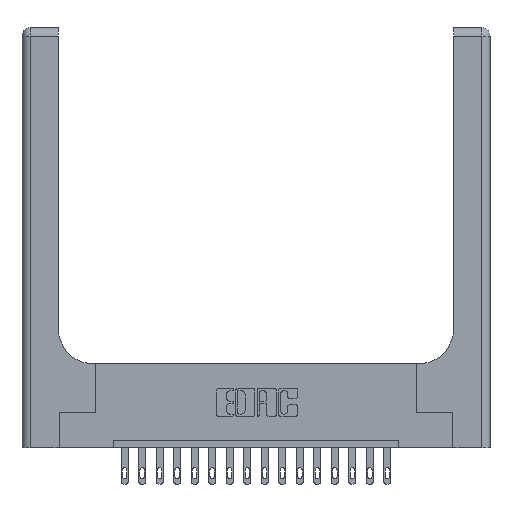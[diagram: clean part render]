
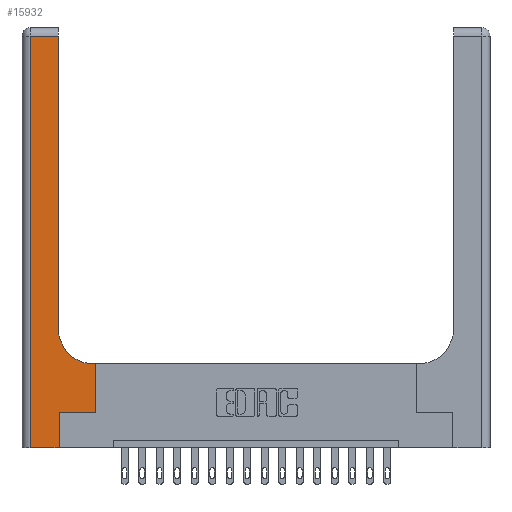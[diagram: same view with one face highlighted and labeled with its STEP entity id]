
A CAD part, top view. The second image highlights one B-rep face of the part: STEP entity #15932.
In plain terms, the highlighted planar face has unit normal (0, 0, 1).
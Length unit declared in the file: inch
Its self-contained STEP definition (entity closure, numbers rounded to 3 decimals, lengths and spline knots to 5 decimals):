
#369 = VERTEX_POINT ( 'NONE', #13812 ) ;
#607 = CARTESIAN_POINT ( 'NONE',  ( 0.265, 0., 0.37 ) ) ;
#915 = VERTEX_POINT ( 'NONE', #9989 ) ;
#1309 = ORIENTED_EDGE ( 'NONE', *, *, #14490, .T. ) ;
#1994 = ORIENTED_EDGE ( 'NONE', *, *, #11978, .T. ) ;
#2414 = CARTESIAN_POINT ( 'NONE',  ( 0., 0., 0.37 ) ) ;
#2613 = VECTOR ( 'NONE', #3500, 39.37008 ) ;
#2908 = CARTESIAN_POINT ( 'NONE',  ( 0.265, 0.25, 0.37 ) ) ;
#2910 = DIRECTION ( 'NONE',  ( -1., 0., 0. ) ) ;
#2995 = VECTOR ( 'NONE', #15745, 39.37008 ) ;
#3332 = VERTEX_POINT ( 'NONE', #2908 ) ;
#3500 = DIRECTION ( 'NONE',  ( 1., 0., 0. ) ) ;
#3819 = LINE ( 'NONE', #12931, #16056 ) ;
#3874 = CARTESIAN_POINT ( 'NONE',  ( 0.26, 3., 0.37 ) ) ;
#4106 = DIRECTION ( 'NONE',  ( 0., -1., 0. ) ) ;
#4144 = CARTESIAN_POINT ( 'NONE',  ( 0.528, 0.6, 0.37 ) ) ;
#4462 = ORIENTED_EDGE ( 'NONE', *, *, #13553, .T. ) ;
#5079 = AXIS2_PLACEMENT_3D ( 'NONE', #10097, #7033, #2910 ) ;
#6234 = CARTESIAN_POINT ( 'NONE',  ( 0., 2.94, 0.37 ) ) ;
#6255 = VERTEX_POINT ( 'NONE', #17951 ) ;
#6872 = VECTOR ( 'NONE', #14143, 39.37008 ) ;
#6894 = LINE ( 'NONE', #12766, #10780 ) ;
#6997 = CARTESIAN_POINT ( 'NONE',  ( 0.06, 2.94, 0.37 ) ) ;
#7033 = DIRECTION ( 'NONE',  ( 0., 0., -1. ) ) ;
#7775 = ORIENTED_EDGE ( 'NONE', *, *, #14515, .T. ) ;
#8270 = CARTESIAN_POINT ( 'NONE',  ( 0.51, 0.85, 0.37 ) ) ;
#8745 = PLANE ( 'NONE',  #5079 ) ;
#8755 = VECTOR ( 'NONE', #15331, 39.37008 ) ;
#8952 = EDGE_CURVE ( 'NONE', #15361, #11487, #13760, .T. ) ;
#9429 = ORIENTED_EDGE ( 'NONE', *, *, #8952, .T. ) ;
#9489 = ORIENTED_EDGE ( 'NONE', *, *, #10337, .T. ) ;
#9832 = CARTESIAN_POINT ( 'NONE',  ( 0.528, 0.25, 0.37 ) ) ;
#9989 = CARTESIAN_POINT ( 'NONE',  ( 0.26, 0.85, 0.37 ) ) ;
#10097 = CARTESIAN_POINT ( 'NONE',  ( 0., 3., 0.37 ) ) ;
#10206 = VECTOR ( 'NONE', #18162, 39.37008 ) ;
#10337 = EDGE_CURVE ( 'NONE', #6255, #14949, #17002, .T. ) ;
#10780 = VECTOR ( 'NONE', #18622, 39.37008 ) ;
#11164 = LINE ( 'NONE', #3874, #6872 ) ;
#11422 = EDGE_CURVE ( 'NONE', #14949, #3332, #18356, .T. ) ;
#11453 = FACE_OUTER_BOUND ( 'NONE', #11567, .T. ) ;
#11487 = VERTEX_POINT ( 'NONE', #4144 ) ;
#11539 = VECTOR ( 'NONE', #14910, 39.37008 ) ;
#11567 = EDGE_LOOP ( 'NONE', ( #7775, #17909, #4462, #9489, #12819, #15950, #9429, #1994, #1309 ) ) ;
#11978 = EDGE_CURVE ( 'NONE', #11487, #369, #6894, .T. ) ;
#12390 = CARTESIAN_POINT ( 'NONE',  ( 0.265, 0., 0.37 ) ) ;
#12766 = CARTESIAN_POINT ( 'NONE',  ( 0.26, 0.6, 0.37 ) ) ;
#12819 = ORIENTED_EDGE ( 'NONE', *, *, #11422, .T. ) ;
#12931 = CARTESIAN_POINT ( 'NONE',  ( 0.06, 3., 0.37 ) ) ;
#13196 = VERTEX_POINT ( 'NONE', #6997 ) ;
#13401 = CARTESIAN_POINT ( 'NONE',  ( 0.265, 0.25, 0.37 ) ) ;
#13539 = LINE ( 'NONE', #6234, #8755 ) ;
#13553 = EDGE_CURVE ( 'NONE', #13196, #6255, #3819, .T. ) ;
#13760 = LINE ( 'NONE', #16727, #11539 ) ;
#13812 = CARTESIAN_POINT ( 'NONE',  ( 0.51, 0.6, 0.37 ) ) ;
#14126 = CARTESIAN_POINT ( 'NONE',  ( 0.26, 2.94, 0.37 ) ) ;
#14143 = DIRECTION ( 'NONE',  ( 0., 1., 0. ) ) ;
#14490 = EDGE_CURVE ( 'NONE', #369, #915, #14844, .T. ) ;
#14515 = EDGE_CURVE ( 'NONE', #915, #16171, #11164, .T. ) ;
#14844 = CIRCLE ( 'NONE', #15157, 0.25 ) ;
#14910 = DIRECTION ( 'NONE',  ( 0., 1., 0. ) ) ;
#14949 = VERTEX_POINT ( 'NONE', #12390 ) ;
#15157 = AXIS2_PLACEMENT_3D ( 'NONE', #8270, #17020, #15485 ) ;
#15331 = DIRECTION ( 'NONE',  ( -1., 0., 0. ) ) ;
#15361 = VERTEX_POINT ( 'NONE', #9832 ) ;
#15485 = DIRECTION ( 'NONE',  ( 1., 0., 0. ) ) ;
#15714 = EDGE_CURVE ( 'NONE', #3332, #15361, #18089, .T. ) ;
#15745 = DIRECTION ( 'NONE',  ( 1., 0., 0. ) ) ;
#15932 = ADVANCED_FACE ( 'NONE', ( #11453 ), #8745, .F. ) ;
#15950 = ORIENTED_EDGE ( 'NONE', *, *, #15714, .T. ) ;
#16056 = VECTOR ( 'NONE', #4106, 39.37008 ) ;
#16171 = VERTEX_POINT ( 'NONE', #14126 ) ;
#16524 = EDGE_CURVE ( 'NONE', #16171, #13196, #13539, .T. ) ;
#16727 = CARTESIAN_POINT ( 'NONE',  ( 0.528, 0.25, 0.37 ) ) ;
#17002 = LINE ( 'NONE', #2414, #2995 ) ;
#17020 = DIRECTION ( 'NONE',  ( 0., 0., -1. ) ) ;
#17909 = ORIENTED_EDGE ( 'NONE', *, *, #16524, .T. ) ;
#17951 = CARTESIAN_POINT ( 'NONE',  ( 0.06, 0., 0.37 ) ) ;
#18089 = LINE ( 'NONE', #13401, #2613 ) ;
#18162 = DIRECTION ( 'NONE',  ( 0., 1., 0. ) ) ;
#18356 = LINE ( 'NONE', #607, #10206 ) ;
#18622 = DIRECTION ( 'NONE',  ( -1., 0., 0. ) ) ;
